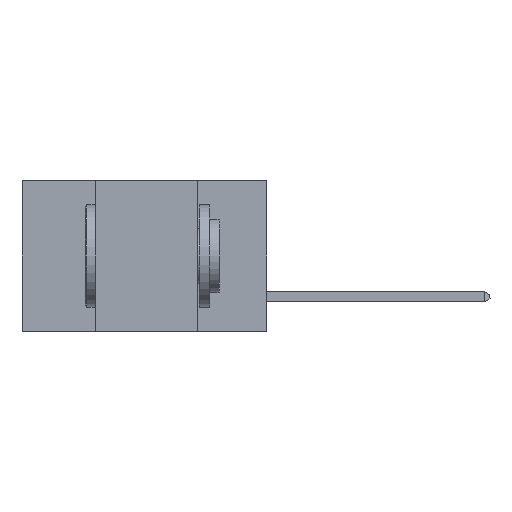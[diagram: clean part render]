
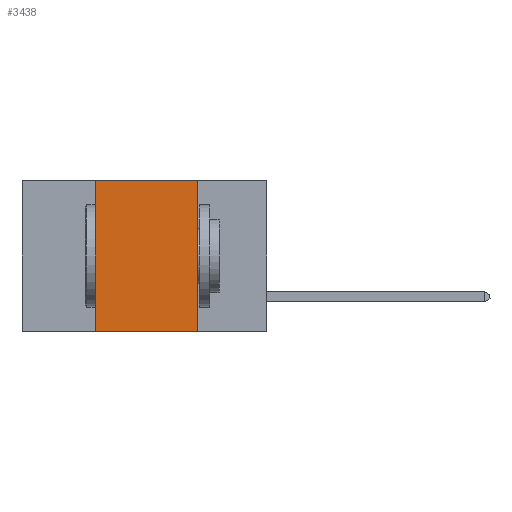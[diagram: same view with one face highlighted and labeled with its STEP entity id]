
A CAD part, left-side view. The second image highlights one B-rep face of the part: STEP entity #3438.
In plain terms, the highlighted planar face has unit normal (-1, 0, 0).
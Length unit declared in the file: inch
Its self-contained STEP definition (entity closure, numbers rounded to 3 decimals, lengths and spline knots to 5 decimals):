
#383 = CARTESIAN_POINT ( 'NONE',  ( 0., 0.17, 0. ) ) ;
#1682 = VERTEX_POINT ( 'NONE', #383 ) ;
#1876 = DIRECTION ( 'NONE',  ( 1., 0., 0. ) ) ;
#1905 = VECTOR ( 'NONE', #4846, 39.37008 ) ;
#1943 = DIRECTION ( 'NONE',  ( 0., 0., -1. ) ) ;
#2074 = PLANE ( 'NONE',  #8872 ) ;
#2390 = EDGE_CURVE ( 'NONE', #3848, #11752, #7896, .T. ) ;
#2595 = CARTESIAN_POINT ( 'NONE',  ( 0., 0.6, 0. ) ) ;
#3181 = DIRECTION ( 'NONE',  ( 0., -1., 0. ) ) ;
#3247 = CARTESIAN_POINT ( 'NONE',  ( 0., 0.42, 0. ) ) ;
#3380 = CARTESIAN_POINT ( 'NONE',  ( 0., 0.42, -0.37 ) ) ;
#3412 = EDGE_CURVE ( 'NONE', #11752, #1682, #10416, .T. ) ;
#3438 = ADVANCED_FACE ( 'NONE', ( #4917 ), #2074, .F. ) ;
#3603 = CARTESIAN_POINT ( 'NONE',  ( 0., 0.6, 0. ) ) ;
#3848 = VERTEX_POINT ( 'NONE', #3380 ) ;
#4435 = LINE ( 'NONE', #10685, #1905 ) ;
#4609 = VECTOR ( 'NONE', #5483, 39.37008 ) ;
#4846 = DIRECTION ( 'NONE',  ( 0., -1., 0. ) ) ;
#4917 = FACE_OUTER_BOUND ( 'NONE', #6811, .T. ) ;
#5343 = VERTEX_POINT ( 'NONE', #8890 ) ;
#5483 = DIRECTION ( 'NONE',  ( 0., 0., -1. ) ) ;
#5558 = VECTOR ( 'NONE', #3181, 39.37008 ) ;
#6811 = EDGE_LOOP ( 'NONE', ( #11545, #9335, #10242, #8289 ) ) ;
#6978 = DIRECTION ( 'NONE',  ( 0., 0., 1. ) ) ;
#7009 = CARTESIAN_POINT ( 'NONE',  ( 0., 0.42, 0. ) ) ;
#7896 = LINE ( 'NONE', #7009, #12610 ) ;
#8289 = ORIENTED_EDGE ( 'NONE', *, *, #10727, .T. ) ;
#8872 = AXIS2_PLACEMENT_3D ( 'NONE', #2595, #1876, #1943 ) ;
#8890 = CARTESIAN_POINT ( 'NONE',  ( 0., 0.17, -0.37 ) ) ;
#9335 = ORIENTED_EDGE ( 'NONE', *, *, #3412, .F. ) ;
#10174 = LINE ( 'NONE', #12184, #4609 ) ;
#10242 = ORIENTED_EDGE ( 'NONE', *, *, #2390, .F. ) ;
#10416 = LINE ( 'NONE', #3603, #5558 ) ;
#10498 = EDGE_CURVE ( 'NONE', #1682, #5343, #10174, .T. ) ;
#10685 = CARTESIAN_POINT ( 'NONE',  ( 0., 0.6, -0.37 ) ) ;
#10727 = EDGE_CURVE ( 'NONE', #3848, #5343, #4435, .T. ) ;
#11545 = ORIENTED_EDGE ( 'NONE', *, *, #10498, .F. ) ;
#11752 = VERTEX_POINT ( 'NONE', #3247 ) ;
#12184 = CARTESIAN_POINT ( 'NONE',  ( 0., 0.17, 0. ) ) ;
#12610 = VECTOR ( 'NONE', #6978, 39.37008 ) ;
